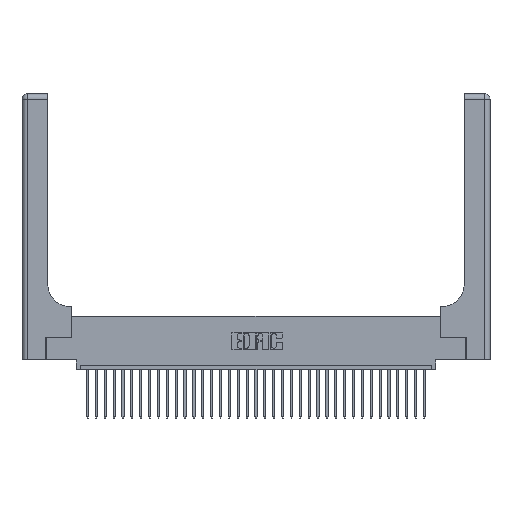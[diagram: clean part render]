
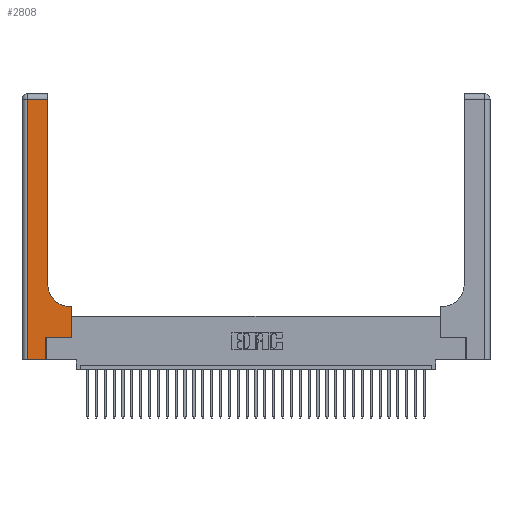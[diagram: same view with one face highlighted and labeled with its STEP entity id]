
A CAD part, top view. The second image highlights one B-rep face of the part: STEP entity #2808.
In plain terms, the highlighted planar face has unit normal (0, 0, 1).
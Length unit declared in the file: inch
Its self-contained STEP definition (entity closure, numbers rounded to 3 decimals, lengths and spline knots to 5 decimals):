
#208 = VECTOR ( 'NONE', #11739, 39.37008 ) ;
#504 = CARTESIAN_POINT ( 'NONE',  ( 0.5585, 0.25, 0.37 ) ) ;
#1152 = DIRECTION ( 'NONE',  ( 0., 1., 0. ) ) ;
#1464 = ORIENTED_EDGE ( 'NONE', *, *, #16222, .T. ) ;
#1474 = EDGE_CURVE ( 'NONE', #7497, #33422, #9538, .T. ) ;
#2000 = DIRECTION ( 'NONE',  ( -1., 0., 0. ) ) ;
#2520 = CARTESIAN_POINT ( 'NONE',  ( 0.2915, 0.85, 0.37 ) ) ;
#2808 = ADVANCED_FACE ( 'NONE', ( #28018 ), #31456, .F. ) ;
#3336 = CARTESIAN_POINT ( 'NONE',  ( 0.06, 2.94, 0.37 ) ) ;
#3677 = DIRECTION ( 'NONE',  ( 0., -1., 0. ) ) ;
#3718 = ORIENTED_EDGE ( 'NONE', *, *, #11802, .T. ) ;
#4987 = VERTEX_POINT ( 'NONE', #3336 ) ;
#5525 = LINE ( 'NONE', #29998, #9324 ) ;
#6060 = AXIS2_PLACEMENT_3D ( 'NONE', #27800, #24706, #24826 ) ;
#6744 = EDGE_CURVE ( 'NONE', #30013, #4987, #8108, .T. ) ;
#7497 = VERTEX_POINT ( 'NONE', #24504 ) ;
#7964 = VECTOR ( 'NONE', #1152, 39.37008 ) ;
#8041 = DIRECTION ( 'NONE',  ( -1., 0., 0. ) ) ;
#8108 = LINE ( 'NONE', #26643, #20325 ) ;
#8731 = DIRECTION ( 'NONE',  ( 1., 0., 0. ) ) ;
#9324 = VECTOR ( 'NONE', #8041, 39.37008 ) ;
#9538 = LINE ( 'NONE', #18587, #30672 ) ;
#9737 = VECTOR ( 'NONE', #17131, 39.37008 ) ;
#9855 = EDGE_CURVE ( 'NONE', #23266, #33210, #10966, .T. ) ;
#10798 = CARTESIAN_POINT ( 'NONE',  ( 0.5585, 0.6, 0.37 ) ) ;
#10966 = LINE ( 'NONE', #504, #9737 ) ;
#11610 = CARTESIAN_POINT ( 'NONE',  ( 0.269, 0., 0.37 ) ) ;
#11734 = CARTESIAN_POINT ( 'NONE',  ( 0.5415, 0.6, 0.37 ) ) ;
#11739 = DIRECTION ( 'NONE',  ( 0., 1., 0. ) ) ;
#11802 = EDGE_CURVE ( 'NONE', #4987, #7497, #32838, .T. ) ;
#12037 = CARTESIAN_POINT ( 'NONE',  ( 0.2915, 3., 0.37 ) ) ;
#12505 = CARTESIAN_POINT ( 'NONE',  ( 0.269, 0.25, 0.37 ) ) ;
#12936 = DIRECTION ( 'NONE',  ( 1., 0., 0. ) ) ;
#13211 = DIRECTION ( 'NONE',  ( -1., 0., 0. ) ) ;
#13275 = AXIS2_PLACEMENT_3D ( 'NONE', #20660, #18179, #2000 ) ;
#13788 = ORIENTED_EDGE ( 'NONE', *, *, #1474, .T. ) ;
#13814 = VECTOR ( 'NONE', #3677, 39.37008 ) ;
#15029 = EDGE_CURVE ( 'NONE', #16257, #30013, #23624, .T. ) ;
#15310 = ORIENTED_EDGE ( 'NONE', *, *, #31460, .T. ) ;
#16222 = EDGE_CURVE ( 'NONE', #33422, #23267, #23530, .T. ) ;
#16257 = VERTEX_POINT ( 'NONE', #2520 ) ;
#17110 = CIRCLE ( 'NONE', #6060, 0.25 ) ;
#17131 = DIRECTION ( 'NONE',  ( 0., 1., 0. ) ) ;
#17577 = LINE ( 'NONE', #18321, #33692 ) ;
#18179 = DIRECTION ( 'NONE',  ( 0., 0., -1. ) ) ;
#18321 = CARTESIAN_POINT ( 'NONE',  ( 0.269, 0.25, 0.37 ) ) ;
#18587 = CARTESIAN_POINT ( 'NONE',  ( 0., 0., 0.37 ) ) ;
#19718 = VERTEX_POINT ( 'NONE', #11734 ) ;
#19862 = CARTESIAN_POINT ( 'NONE',  ( 0.06, 3., 0.37 ) ) ;
#20325 = VECTOR ( 'NONE', #13211, 39.37008 ) ;
#20660 = CARTESIAN_POINT ( 'NONE',  ( 0., 3., 0.37 ) ) ;
#23266 = VERTEX_POINT ( 'NONE', #33909 ) ;
#23267 = VERTEX_POINT ( 'NONE', #12505 ) ;
#23530 = LINE ( 'NONE', #11610, #208 ) ;
#23624 = LINE ( 'NONE', #12037, #7964 ) ;
#23948 = ORIENTED_EDGE ( 'NONE', *, *, #6744, .T. ) ;
#24079 = CARTESIAN_POINT ( 'NONE',  ( 0.2915, 2.94, 0.37 ) ) ;
#24504 = CARTESIAN_POINT ( 'NONE',  ( 0.06, 0., 0.37 ) ) ;
#24706 = DIRECTION ( 'NONE',  ( 0., 0., -1. ) ) ;
#24826 = DIRECTION ( 'NONE',  ( 1., 0., 0. ) ) ;
#25027 = CARTESIAN_POINT ( 'NONE',  ( 0.269, 0., 0.37 ) ) ;
#26192 = ORIENTED_EDGE ( 'NONE', *, *, #28916, .T. ) ;
#26643 = CARTESIAN_POINT ( 'NONE',  ( 0., 2.94, 0.37 ) ) ;
#27634 = EDGE_LOOP ( 'NONE', ( #29843, #23948, #3718, #13788, #1464, #28122, #35059, #15310, #26192 ) ) ;
#27800 = CARTESIAN_POINT ( 'NONE',  ( 0.5415, 0.85, 0.37 ) ) ;
#28018 = FACE_OUTER_BOUND ( 'NONE', #27634, .T. ) ;
#28122 = ORIENTED_EDGE ( 'NONE', *, *, #33594, .T. ) ;
#28916 = EDGE_CURVE ( 'NONE', #19718, #16257, #17110, .T. ) ;
#29843 = ORIENTED_EDGE ( 'NONE', *, *, #15029, .T. ) ;
#29998 = CARTESIAN_POINT ( 'NONE',  ( 0.2915, 0.6, 0.37 ) ) ;
#30013 = VERTEX_POINT ( 'NONE', #24079 ) ;
#30672 = VECTOR ( 'NONE', #8731, 39.37008 ) ;
#31456 = PLANE ( 'NONE',  #13275 ) ;
#31460 = EDGE_CURVE ( 'NONE', #33210, #19718, #5525, .T. ) ;
#32838 = LINE ( 'NONE', #19862, #13814 ) ;
#33210 = VERTEX_POINT ( 'NONE', #10798 ) ;
#33422 = VERTEX_POINT ( 'NONE', #25027 ) ;
#33594 = EDGE_CURVE ( 'NONE', #23267, #23266, #17577, .T. ) ;
#33692 = VECTOR ( 'NONE', #12936, 39.37008 ) ;
#33909 = CARTESIAN_POINT ( 'NONE',  ( 0.5585, 0.25, 0.37 ) ) ;
#35059 = ORIENTED_EDGE ( 'NONE', *, *, #9855, .T. ) ;
